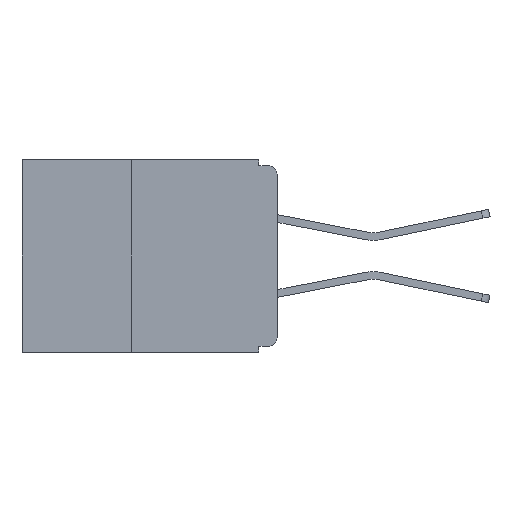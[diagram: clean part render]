
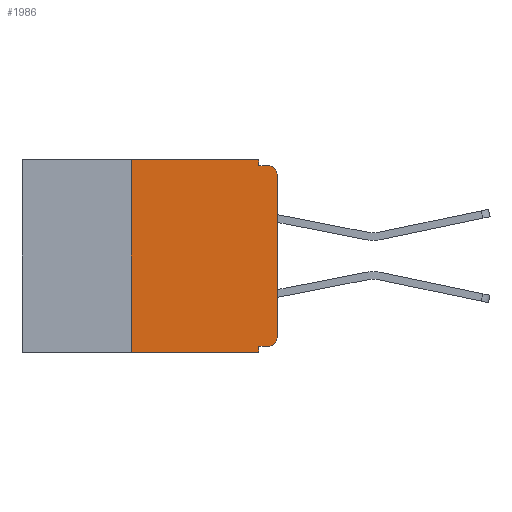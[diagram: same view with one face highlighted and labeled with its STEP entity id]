
A CAD part, left-side view. The second image highlights one B-rep face of the part: STEP entity #1986.
In plain terms, the highlighted planar face has unit normal (-1, 0, 0).
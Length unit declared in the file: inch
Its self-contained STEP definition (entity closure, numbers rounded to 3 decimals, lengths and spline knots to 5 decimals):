
#148 = VERTEX_POINT ( 'NONE', #19974 ) ;
#649 = CARTESIAN_POINT ( 'NONE',  ( 0., 0., -0.305 ) ) ;
#694 = EDGE_CURVE ( 'NONE', #9096, #28231, #3929, .T. ) ;
#907 = ORIENTED_EDGE ( 'NONE', *, *, #29113, .T. ) ;
#963 = VERTEX_POINT ( 'NONE', #12133 ) ;
#1288 = VECTOR ( 'NONE', #18322, 39.37008 ) ;
#1556 = CARTESIAN_POINT ( 'NONE',  ( 0., 0.031, 0. ) ) ;
#1938 = DIRECTION ( 'NONE',  ( 1., 0., 0. ) ) ;
#1986 = ADVANCED_FACE ( 'NONE', ( #5353 ), #8306, .F. ) ;
#2547 = DIRECTION ( 'NONE',  ( -1., 0., 0. ) ) ;
#2553 = EDGE_LOOP ( 'NONE', ( #21946, #13108, #5471, #4206, #21320, #13713, #907, #19664, #6602, #14429 ) ) ;
#2623 = DIRECTION ( 'NONE',  ( 0., 0., -1. ) ) ;
#2826 = LINE ( 'NONE', #27838, #27848 ) ;
#3065 = VERTEX_POINT ( 'NONE', #10206 ) ;
#3232 = EDGE_CURVE ( 'NONE', #963, #148, #10513, .T. ) ;
#3377 = EDGE_CURVE ( 'NONE', #19779, #963, #26212, .T. ) ;
#3929 = LINE ( 'NONE', #18232, #26722 ) ;
#4206 = ORIENTED_EDGE ( 'NONE', *, *, #5025, .F. ) ;
#4648 = EDGE_CURVE ( 'NONE', #5455, #3065, #5565, .T. ) ;
#4819 = VECTOR ( 'NONE', #16981, 39.37008 ) ;
#5025 = EDGE_CURVE ( 'NONE', #148, #23439, #19628, .T. ) ;
#5269 = EDGE_CURVE ( 'NONE', #5455, #9096, #6652, .T. ) ;
#5353 = FACE_OUTER_BOUND ( 'NONE', #2553, .T. ) ;
#5455 = VERTEX_POINT ( 'NONE', #26748 ) ;
#5471 = ORIENTED_EDGE ( 'NONE', *, *, #15829, .F. ) ;
#5524 = AXIS2_PLACEMENT_3D ( 'NONE', #24166, #10141, #26470 ) ;
#5565 = LINE ( 'NONE', #16690, #4819 ) ;
#6602 = ORIENTED_EDGE ( 'NONE', *, *, #4648, .F. ) ;
#6652 = CIRCLE ( 'NONE', #11600, 0.015 ) ;
#7574 = VECTOR ( 'NONE', #24467, 39.37008 ) ;
#8306 = PLANE ( 'NONE',  #24858 ) ;
#9052 = CARTESIAN_POINT ( 'NONE',  ( 0., 0.031, -0.01 ) ) ;
#9068 = CARTESIAN_POINT ( 'NONE',  ( 0., 0.031, -0.33 ) ) ;
#9096 = VERTEX_POINT ( 'NONE', #649 ) ;
#9099 = LINE ( 'NONE', #15105, #7574 ) ;
#10141 = DIRECTION ( 'NONE',  ( -1., 0., 0. ) ) ;
#10206 = CARTESIAN_POINT ( 'NONE',  ( 0., 0.031, -0.32 ) ) ;
#10266 = CARTESIAN_POINT ( 'NONE',  ( 0., 0.031, -0.33 ) ) ;
#10400 = VERTEX_POINT ( 'NONE', #27499 ) ;
#10513 = LINE ( 'NONE', #23640, #16804 ) ;
#11555 = DIRECTION ( 'NONE',  ( 0., -1., 0. ) ) ;
#11600 = AXIS2_PLACEMENT_3D ( 'NONE', #16850, #2547, #19213 ) ;
#11723 = VERTEX_POINT ( 'NONE', #9068 ) ;
#12133 = CARTESIAN_POINT ( 'NONE',  ( 0., 0.25, 0. ) ) ;
#12242 = DIRECTION ( 'NONE',  ( 0., 0., 1. ) ) ;
#12611 = DIRECTION ( 'NONE',  ( 0., 0., -1. ) ) ;
#13108 = ORIENTED_EDGE ( 'NONE', *, *, #28790, .T. ) ;
#13713 = ORIENTED_EDGE ( 'NONE', *, *, #3377, .F. ) ;
#14429 = ORIENTED_EDGE ( 'NONE', *, *, #5269, .T. ) ;
#15105 = CARTESIAN_POINT ( 'NONE',  ( 0., 0., -0.01 ) ) ;
#15829 = EDGE_CURVE ( 'NONE', #23439, #10400, #9099, .T. ) ;
#16690 = CARTESIAN_POINT ( 'NONE',  ( 0., 0., -0.32 ) ) ;
#16804 = VECTOR ( 'NONE', #23544, 39.37008 ) ;
#16850 = CARTESIAN_POINT ( 'NONE',  ( 0., 0.015, -0.305 ) ) ;
#16981 = DIRECTION ( 'NONE',  ( 0., 1., 0. ) ) ;
#18232 = CARTESIAN_POINT ( 'NONE',  ( 0., 0., 0. ) ) ;
#18322 = DIRECTION ( 'NONE',  ( 0., 0., -1. ) ) ;
#18795 = DIRECTION ( 'NONE',  ( 0., 0., 1. ) ) ;
#19041 = CARTESIAN_POINT ( 'NONE',  ( 0., 0.25, -0.33 ) ) ;
#19213 = DIRECTION ( 'NONE',  ( 0., 0., -1. ) ) ;
#19615 = CIRCLE ( 'NONE', #5524, 0.015 ) ;
#19628 = LINE ( 'NONE', #1556, #1288 ) ;
#19664 = ORIENTED_EDGE ( 'NONE', *, *, #27609, .F. ) ;
#19779 = VERTEX_POINT ( 'NONE', #25981 ) ;
#19974 = CARTESIAN_POINT ( 'NONE',  ( 0., 0.031, 0. ) ) ;
#21097 = LINE ( 'NONE', #10266, #26482 ) ;
#21320 = ORIENTED_EDGE ( 'NONE', *, *, #3232, .F. ) ;
#21946 = ORIENTED_EDGE ( 'NONE', *, *, #694, .T. ) ;
#23439 = VERTEX_POINT ( 'NONE', #9052 ) ;
#23544 = DIRECTION ( 'NONE',  ( 0., -1., 0. ) ) ;
#23640 = CARTESIAN_POINT ( 'NONE',  ( 0., 0.437, 0. ) ) ;
#23795 = CARTESIAN_POINT ( 'NONE',  ( 0., 0., -0.025 ) ) ;
#24166 = CARTESIAN_POINT ( 'NONE',  ( 0., 0.015, -0.025 ) ) ;
#24467 = DIRECTION ( 'NONE',  ( 0., -1., 0. ) ) ;
#24777 = VECTOR ( 'NONE', #18795, 39.37008 ) ;
#24858 = AXIS2_PLACEMENT_3D ( 'NONE', #25844, #1938, #2623 ) ;
#25844 = CARTESIAN_POINT ( 'NONE',  ( 0., 0.437, 0. ) ) ;
#25981 = CARTESIAN_POINT ( 'NONE',  ( 0., 0.25, -0.33 ) ) ;
#26212 = LINE ( 'NONE', #19041, #24777 ) ;
#26470 = DIRECTION ( 'NONE',  ( 0., 0., -1. ) ) ;
#26482 = VECTOR ( 'NONE', #12611, 39.37008 ) ;
#26722 = VECTOR ( 'NONE', #12242, 39.37008 ) ;
#26748 = CARTESIAN_POINT ( 'NONE',  ( 0., 0.015, -0.32 ) ) ;
#27499 = CARTESIAN_POINT ( 'NONE',  ( 0., 0.015, -0.01 ) ) ;
#27609 = EDGE_CURVE ( 'NONE', #3065, #11723, #21097, .T. ) ;
#27838 = CARTESIAN_POINT ( 'NONE',  ( 0., 0.437, -0.33 ) ) ;
#27848 = VECTOR ( 'NONE', #11555, 39.37008 ) ;
#28231 = VERTEX_POINT ( 'NONE', #23795 ) ;
#28790 = EDGE_CURVE ( 'NONE', #28231, #10400, #19615, .T. ) ;
#29113 = EDGE_CURVE ( 'NONE', #19779, #11723, #2826, .T. ) ;
